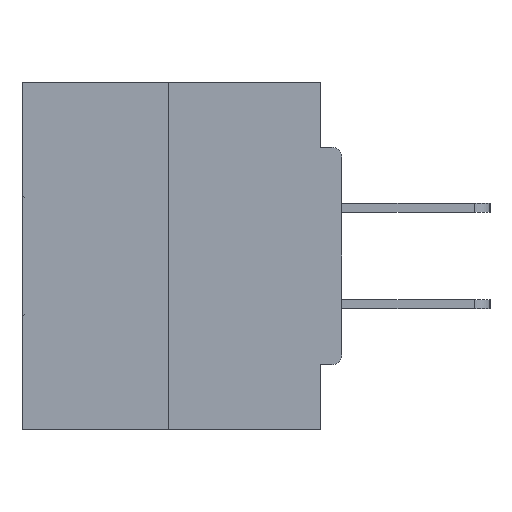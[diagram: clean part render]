
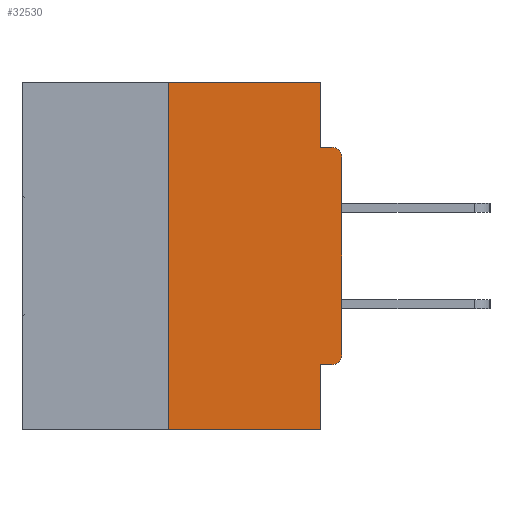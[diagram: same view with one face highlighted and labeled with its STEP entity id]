
A CAD part, left-side view. The second image highlights one B-rep face of the part: STEP entity #32530.
In plain terms, the highlighted planar face has unit normal (-1, 0, 0).
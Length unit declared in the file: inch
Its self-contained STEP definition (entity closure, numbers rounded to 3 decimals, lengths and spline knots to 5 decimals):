
#1564 = VERTEX_POINT ( 'NONE', #14509 ) ;
#2312 = FACE_OUTER_BOUND ( 'NONE', #36927, .T. ) ;
#2327 = CARTESIAN_POINT ( 'NONE',  ( 0., 0.25, 0. ) ) ;
#2531 = VERTEX_POINT ( 'NONE', #39677 ) ;
#2656 = DIRECTION ( 'NONE',  ( 0., -1., 0. ) ) ;
#2900 = LINE ( 'NONE', #14711, #34735 ) ;
#3379 = EDGE_CURVE ( 'NONE', #28454, #4956, #11103, .T. ) ;
#4502 = CARTESIAN_POINT ( 'NONE',  ( 0., 0.25, 0. ) ) ;
#4516 = LINE ( 'NONE', #9373, #22365 ) ;
#4597 = LINE ( 'NONE', #30408, #33554 ) ;
#4683 = ORIENTED_EDGE ( 'NONE', *, *, #36563, .F. ) ;
#4725 = CIRCLE ( 'NONE', #13237, 0.015 ) ;
#4956 = VERTEX_POINT ( 'NONE', #23855 ) ;
#5333 = CARTESIAN_POINT ( 'NONE',  ( 0., 0.015, -0.4065 ) ) ;
#5630 = CARTESIAN_POINT ( 'NONE',  ( 0., 0., -0.3915 ) ) ;
#5634 = LINE ( 'NONE', #21066, #7061 ) ;
#7061 = VECTOR ( 'NONE', #2656, 39.37008 ) ;
#7387 = PLANE ( 'NONE',  #36051 ) ;
#8193 = DIRECTION ( 'NONE',  ( 0., 0., 1. ) ) ;
#8197 = ORIENTED_EDGE ( 'NONE', *, *, #37076, .F. ) ;
#9116 = DIRECTION ( 'NONE',  ( 0., 1., 0. ) ) ;
#9373 = CARTESIAN_POINT ( 'NONE',  ( 0., 0.031, 0. ) ) ;
#9944 = VECTOR ( 'NONE', #36702, 39.37008 ) ;
#10391 = VERTEX_POINT ( 'NONE', #35635 ) ;
#10902 = LINE ( 'NONE', #12093, #9944 ) ;
#11103 = LINE ( 'NONE', #33973, #33823 ) ;
#11267 = LINE ( 'NONE', #2327, #33026 ) ;
#11881 = DIRECTION ( 'NONE',  ( 0., -1., 0. ) ) ;
#12093 = CARTESIAN_POINT ( 'NONE',  ( 0., 0.031, -0.5 ) ) ;
#12140 = CARTESIAN_POINT ( 'NONE',  ( 0., 0.015, -0.1085 ) ) ;
#12195 = CARTESIAN_POINT ( 'NONE',  ( 0., 0.031, -0.5 ) ) ;
#12225 = VERTEX_POINT ( 'NONE', #31139 ) ;
#12437 = EDGE_CURVE ( 'NONE', #4956, #29597, #10902, .T. ) ;
#12750 = VERTEX_POINT ( 'NONE', #5630 ) ;
#13237 = AXIS2_PLACEMENT_3D ( 'NONE', #12140, #21419, #37293 ) ;
#13979 = DIRECTION ( 'NONE',  ( 0., 0., -1. ) ) ;
#14509 = CARTESIAN_POINT ( 'NONE',  ( 0., 0.015, -0.0935 ) ) ;
#14711 = CARTESIAN_POINT ( 'NONE',  ( 0., 0.46, -0.5 ) ) ;
#16241 = DIRECTION ( 'NONE',  ( -1., 0., 0. ) ) ;
#16335 = EDGE_CURVE ( 'NONE', #12225, #29597, #2900, .T. ) ;
#17418 = ORIENTED_EDGE ( 'NONE', *, *, #37256, .F. ) ;
#18642 = ORIENTED_EDGE ( 'NONE', *, *, #16335, .T. ) ;
#19177 = LINE ( 'NONE', #24915, #38103 ) ;
#19460 = VERTEX_POINT ( 'NONE', #4502 ) ;
#20065 = CARTESIAN_POINT ( 'NONE',  ( 0., 0.46, 0. ) ) ;
#21066 = CARTESIAN_POINT ( 'NONE',  ( 0., 0.46, 0. ) ) ;
#21419 = DIRECTION ( 'NONE',  ( -1., 0., 0. ) ) ;
#21858 = CARTESIAN_POINT ( 'NONE',  ( 0., 0., -0.1085 ) ) ;
#22365 = VECTOR ( 'NONE', #31121, 39.37008 ) ;
#22819 = ORIENTED_EDGE ( 'NONE', *, *, #30442, .T. ) ;
#23313 = DIRECTION ( 'NONE',  ( 1., 0., 0. ) ) ;
#23522 = DIRECTION ( 'NONE',  ( 0., -1., 0. ) ) ;
#23855 = CARTESIAN_POINT ( 'NONE',  ( 0., 0.031, -0.4065 ) ) ;
#24218 = ORIENTED_EDGE ( 'NONE', *, *, #31382, .F. ) ;
#24915 = CARTESIAN_POINT ( 'NONE',  ( 0., 0., 0. ) ) ;
#25823 = DIRECTION ( 'NONE',  ( 0., 0., 1. ) ) ;
#27693 = ORIENTED_EDGE ( 'NONE', *, *, #3379, .F. ) ;
#28454 = VERTEX_POINT ( 'NONE', #5333 ) ;
#29160 = VERTEX_POINT ( 'NONE', #21858 ) ;
#29536 = ORIENTED_EDGE ( 'NONE', *, *, #32469, .T. ) ;
#29597 = VERTEX_POINT ( 'NONE', #12195 ) ;
#30387 = EDGE_CURVE ( 'NONE', #12750, #29160, #19177, .T. ) ;
#30408 = CARTESIAN_POINT ( 'NONE',  ( 0., 0., -0.0935 ) ) ;
#30442 = EDGE_CURVE ( 'NONE', #28454, #12750, #35151, .T. ) ;
#31121 = DIRECTION ( 'NONE',  ( 0., 0., -1. ) ) ;
#31139 = CARTESIAN_POINT ( 'NONE',  ( 0., 0.25, -0.5 ) ) ;
#31382 = EDGE_CURVE ( 'NONE', #19460, #10391, #5634, .T. ) ;
#31949 = DIRECTION ( 'NONE',  ( 0., 0., -1. ) ) ;
#32469 = EDGE_CURVE ( 'NONE', #29160, #1564, #4725, .T. ) ;
#32530 = ADVANCED_FACE ( 'NONE', ( #2312 ), #7387, .F. ) ;
#32853 = ORIENTED_EDGE ( 'NONE', *, *, #12437, .F. ) ;
#33026 = VECTOR ( 'NONE', #8193, 39.37008 ) ;
#33554 = VECTOR ( 'NONE', #11881, 39.37008 ) ;
#33823 = VECTOR ( 'NONE', #9116, 39.37008 ) ;
#33973 = CARTESIAN_POINT ( 'NONE',  ( 0., 0., -0.4065 ) ) ;
#34735 = VECTOR ( 'NONE', #23522, 39.37008 ) ;
#35151 = CIRCLE ( 'NONE', #39412, 0.015 ) ;
#35406 = ORIENTED_EDGE ( 'NONE', *, *, #30387, .T. ) ;
#35635 = CARTESIAN_POINT ( 'NONE',  ( 0., 0.031, 0. ) ) ;
#36051 = AXIS2_PLACEMENT_3D ( 'NONE', #20065, #23313, #13979 ) ;
#36563 = EDGE_CURVE ( 'NONE', #2531, #1564, #4597, .T. ) ;
#36702 = DIRECTION ( 'NONE',  ( 0., 0., -1. ) ) ;
#36927 = EDGE_LOOP ( 'NONE', ( #24218, #8197, #18642, #32853, #27693, #22819, #35406, #29536, #4683, #17418 ) ) ;
#37076 = EDGE_CURVE ( 'NONE', #12225, #19460, #11267, .T. ) ;
#37256 = EDGE_CURVE ( 'NONE', #10391, #2531, #4516, .T. ) ;
#37293 = DIRECTION ( 'NONE',  ( 0., 0., -1. ) ) ;
#38103 = VECTOR ( 'NONE', #25823, 39.37008 ) ;
#38318 = CARTESIAN_POINT ( 'NONE',  ( 0., 0.015, -0.3915 ) ) ;
#39412 = AXIS2_PLACEMENT_3D ( 'NONE', #38318, #16241, #31949 ) ;
#39677 = CARTESIAN_POINT ( 'NONE',  ( 0., 0.031, -0.0935 ) ) ;
